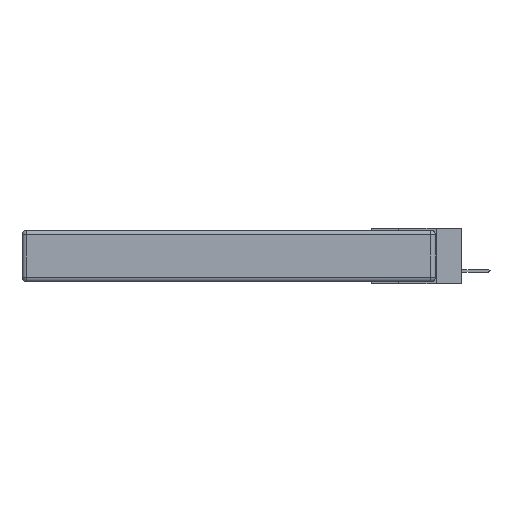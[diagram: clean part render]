
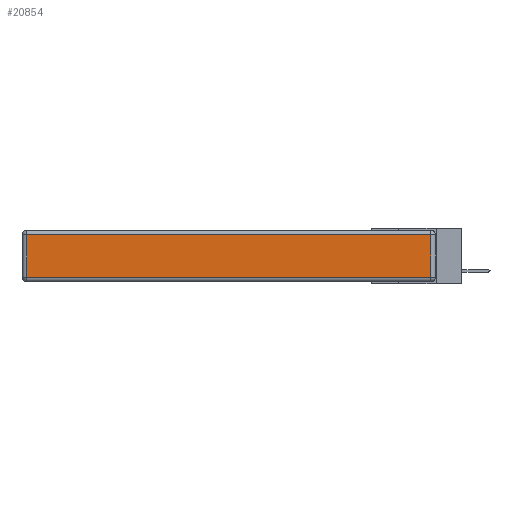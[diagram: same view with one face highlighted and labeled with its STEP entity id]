
A CAD part, left-side view. The second image highlights one B-rep face of the part: STEP entity #20854.
In plain terms, the highlighted planar face has unit normal (-1, 0, 0).
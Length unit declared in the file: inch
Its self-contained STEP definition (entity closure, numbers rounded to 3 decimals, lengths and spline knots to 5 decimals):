
#1181 = DIRECTION ( 'NONE',  ( 0., 0., 1. ) ) ;
#1370 = ORIENTED_EDGE ( 'NONE', *, *, #13733, .T. ) ;
#3609 = EDGE_CURVE ( 'NONE', #13196, #11837, #4530, .T. ) ;
#3780 = CARTESIAN_POINT ( 'NONE',  ( 0., 2.72, -0.313 ) ) ;
#4383 = LINE ( 'NONE', #14868, #23197 ) ;
#4530 = LINE ( 'NONE', #11696, #20337 ) ;
#5153 = DIRECTION ( 'NONE',  ( 0., 0., 1. ) ) ;
#6576 = EDGE_CURVE ( 'NONE', #28074, #21323, #4383, .T. ) ;
#6720 = DIRECTION ( 'NONE',  ( 0., 0., -1. ) ) ;
#8263 = DIRECTION ( 'NONE',  ( 0., 1., 0. ) ) ;
#9754 = ORIENTED_EDGE ( 'NONE', *, *, #3609, .T. ) ;
#11696 = CARTESIAN_POINT ( 'NONE',  ( 0., 2.72, -0.343 ) ) ;
#11837 = VERTEX_POINT ( 'NONE', #3780 ) ;
#12772 = LINE ( 'NONE', #13511, #21779 ) ;
#12891 = CARTESIAN_POINT ( 'NONE',  ( 0., 0., -0.343 ) ) ;
#13196 = VERTEX_POINT ( 'NONE', #15763 ) ;
#13511 = CARTESIAN_POINT ( 'NONE',  ( 0., 0., -0.313 ) ) ;
#13733 = EDGE_CURVE ( 'NONE', #21323, #13196, #29107, .T. ) ;
#14868 = CARTESIAN_POINT ( 'NONE',  ( 0., 0.03, -0.343 ) ) ;
#15009 = ORIENTED_EDGE ( 'NONE', *, *, #26374, .T. ) ;
#15552 = CARTESIAN_POINT ( 'NONE',  ( 0., 0.03, -0.313 ) ) ;
#15763 = CARTESIAN_POINT ( 'NONE',  ( 0., 2.72, -0.03 ) ) ;
#16331 = EDGE_LOOP ( 'NONE', ( #15009, #18758, #1370, #9754 ) ) ;
#16352 = VECTOR ( 'NONE', #8263, 39.37008 ) ;
#17806 = DIRECTION ( 'NONE',  ( -1., 0., 0. ) ) ;
#18758 = ORIENTED_EDGE ( 'NONE', *, *, #6576, .T. ) ;
#20220 = DIRECTION ( 'NONE',  ( 0., -1., 0. ) ) ;
#20239 = CARTESIAN_POINT ( 'NONE',  ( 0., 2.75, -0.03 ) ) ;
#20337 = VECTOR ( 'NONE', #6720, 39.37008 ) ;
#20854 = ADVANCED_FACE ( 'NONE', ( #30713 ), #26962, .T. ) ;
#21323 = VERTEX_POINT ( 'NONE', #30702 ) ;
#21779 = VECTOR ( 'NONE', #20220, 39.37008 ) ;
#23197 = VECTOR ( 'NONE', #5153, 39.37008 ) ;
#26374 = EDGE_CURVE ( 'NONE', #11837, #28074, #12772, .T. ) ;
#26962 = PLANE ( 'NONE',  #28393 ) ;
#28074 = VERTEX_POINT ( 'NONE', #15552 ) ;
#28393 = AXIS2_PLACEMENT_3D ( 'NONE', #12891, #17806, #1181 ) ;
#29107 = LINE ( 'NONE', #20239, #16352 ) ;
#30702 = CARTESIAN_POINT ( 'NONE',  ( 0., 0.03, -0.03 ) ) ;
#30713 = FACE_OUTER_BOUND ( 'NONE', #16331, .T. ) ;
